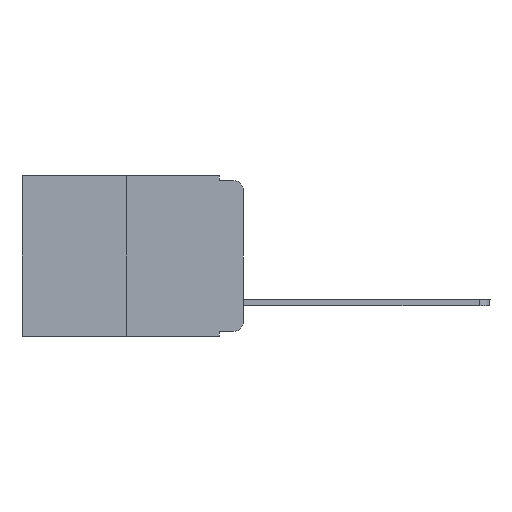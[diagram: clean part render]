
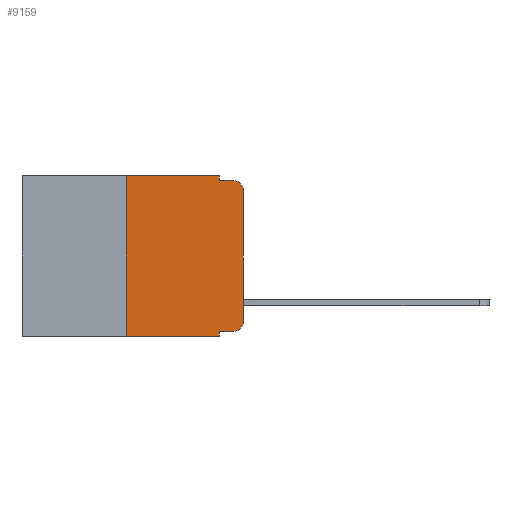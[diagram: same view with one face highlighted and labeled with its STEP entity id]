
A CAD part, left-side view. The second image highlights one B-rep face of the part: STEP entity #9159.
In plain terms, the highlighted planar face has unit normal (-1, 0, 0).
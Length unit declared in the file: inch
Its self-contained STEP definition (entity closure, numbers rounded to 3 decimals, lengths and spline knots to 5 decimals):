
#197 = LINE ( 'NONE', #9961, #6033 ) ;
#216 = DIRECTION ( 'NONE',  ( 0., 0., 1. ) ) ;
#510 = EDGE_CURVE ( 'NONE', #4199, #9617, #7737, .T. ) ;
#622 = PLANE ( 'NONE',  #2377 ) ;
#712 = CIRCLE ( 'NONE', #5788, 0.02 ) ;
#832 = CARTESIAN_POINT ( 'NONE',  ( 0., 0.473, 0. ) ) ;
#838 = LINE ( 'NONE', #6818, #10689 ) ;
#858 = DIRECTION ( 'NONE',  ( 0., -1., 0. ) ) ;
#878 = VECTOR ( 'NONE', #5546, 39.37008 ) ;
#1097 = EDGE_CURVE ( 'NONE', #9617, #4629, #4163, .T. ) ;
#1156 = CARTESIAN_POINT ( 'NONE',  ( 0., 0.02, -0.313 ) ) ;
#1245 = VECTOR ( 'NONE', #9817, 39.37008 ) ;
#1363 = DIRECTION ( 'NONE',  ( 0., 0., -1. ) ) ;
#1670 = DIRECTION ( 'NONE',  ( -1., 0., 0. ) ) ;
#2124 = EDGE_CURVE ( 'NONE', #9114, #5844, #5561, .T. ) ;
#2151 = CARTESIAN_POINT ( 'NONE',  ( 0., 0.051, -0.333 ) ) ;
#2206 = ORIENTED_EDGE ( 'NONE', *, *, #2124, .T. ) ;
#2251 = CARTESIAN_POINT ( 'NONE',  ( 0., 0.051, 0. ) ) ;
#2377 = AXIS2_PLACEMENT_3D ( 'NONE', #10420, #6311, #1363 ) ;
#2617 = ORIENTED_EDGE ( 'NONE', *, *, #9771, .T. ) ;
#2679 = CARTESIAN_POINT ( 'NONE',  ( 0., 0., -0.313 ) ) ;
#2784 = ORIENTED_EDGE ( 'NONE', *, *, #6930, .F. ) ;
#3306 = LINE ( 'NONE', #8320, #6009 ) ;
#3744 = DIRECTION ( 'NONE',  ( -1., 0., 0. ) ) ;
#4052 = ORIENTED_EDGE ( 'NONE', *, *, #8165, .T. ) ;
#4053 = VECTOR ( 'NONE', #10527, 39.37008 ) ;
#4152 = VECTOR ( 'NONE', #4890, 39.37008 ) ;
#4163 = LINE ( 'NONE', #9756, #4152 ) ;
#4199 = VERTEX_POINT ( 'NONE', #8731 ) ;
#4396 = ORIENTED_EDGE ( 'NONE', *, *, #1097, .F. ) ;
#4552 = ORIENTED_EDGE ( 'NONE', *, *, #9254, .F. ) ;
#4629 = VERTEX_POINT ( 'NONE', #7718 ) ;
#4722 = CARTESIAN_POINT ( 'NONE',  ( 0., 0.25, -0.343 ) ) ;
#4819 = CARTESIAN_POINT ( 'NONE',  ( 0., 0., -0.03 ) ) ;
#4890 = DIRECTION ( 'NONE',  ( 0., 0., -1. ) ) ;
#4948 = ORIENTED_EDGE ( 'NONE', *, *, #8625, .F. ) ;
#5010 = CARTESIAN_POINT ( 'NONE',  ( 0., 0.02, -0.03 ) ) ;
#5152 = DIRECTION ( 'NONE',  ( 0., -1., 0. ) ) ;
#5404 = VECTOR ( 'NONE', #5794, 39.37008 ) ;
#5480 = EDGE_CURVE ( 'NONE', #8730, #5530, #3306, .T. ) ;
#5530 = VERTEX_POINT ( 'NONE', #10038 ) ;
#5546 = DIRECTION ( 'NONE',  ( 0., 0., 1. ) ) ;
#5561 = LINE ( 'NONE', #7059, #878 ) ;
#5788 = AXIS2_PLACEMENT_3D ( 'NONE', #5010, #1670, #9972 ) ;
#5794 = DIRECTION ( 'NONE',  ( 0., -1., 0. ) ) ;
#5824 = ORIENTED_EDGE ( 'NONE', *, *, #9613, .T. ) ;
#5844 = VERTEX_POINT ( 'NONE', #4819 ) ;
#6009 = VECTOR ( 'NONE', #5152, 39.37008 ) ;
#6033 = VECTOR ( 'NONE', #858, 39.37008 ) ;
#6241 = ORIENTED_EDGE ( 'NONE', *, *, #510, .F. ) ;
#6311 = DIRECTION ( 'NONE',  ( 1., 0., 0. ) ) ;
#6318 = CARTESIAN_POINT ( 'NONE',  ( 0., 0.473, -0.343 ) ) ;
#6320 = CARTESIAN_POINT ( 'NONE',  ( 0., 0.02, -0.01 ) ) ;
#6750 = EDGE_LOOP ( 'NONE', ( #2206, #5824, #4552, #4396, #6241, #4948, #4052, #2784, #6813, #2617 ) ) ;
#6791 = LINE ( 'NONE', #2251, #4053 ) ;
#6813 = ORIENTED_EDGE ( 'NONE', *, *, #5480, .T. ) ;
#6818 = CARTESIAN_POINT ( 'NONE',  ( 0., 0.25, 0. ) ) ;
#6930 = EDGE_CURVE ( 'NONE', #8730, #8749, #6791, .T. ) ;
#6940 = FACE_OUTER_BOUND ( 'NONE', #6750, .T. ) ;
#7059 = CARTESIAN_POINT ( 'NONE',  ( 0., 0., 0. ) ) ;
#7466 = LINE ( 'NONE', #6318, #1245 ) ;
#7718 = CARTESIAN_POINT ( 'NONE',  ( 0., 0.051, -0.01 ) ) ;
#7737 = LINE ( 'NONE', #832, #5404 ) ;
#7952 = CARTESIAN_POINT ( 'NONE',  ( 0., 0.051, -0.343 ) ) ;
#8165 = EDGE_CURVE ( 'NONE', #10624, #8749, #7466, .T. ) ;
#8320 = CARTESIAN_POINT ( 'NONE',  ( 0., 0.051, -0.333 ) ) ;
#8625 = EDGE_CURVE ( 'NONE', #10624, #4199, #838, .T. ) ;
#8680 = VERTEX_POINT ( 'NONE', #6320 ) ;
#8730 = VERTEX_POINT ( 'NONE', #2151 ) ;
#8731 = CARTESIAN_POINT ( 'NONE',  ( 0., 0.25, 0. ) ) ;
#8749 = VERTEX_POINT ( 'NONE', #7952 ) ;
#9114 = VERTEX_POINT ( 'NONE', #2679 ) ;
#9135 = CARTESIAN_POINT ( 'NONE',  ( 0., 0.051, 0. ) ) ;
#9159 = ADVANCED_FACE ( 'NONE', ( #6940 ), #622, .F. ) ;
#9254 = EDGE_CURVE ( 'NONE', #4629, #8680, #197, .T. ) ;
#9507 = DIRECTION ( 'NONE',  ( 0., 0., -1. ) ) ;
#9613 = EDGE_CURVE ( 'NONE', #5844, #8680, #712, .T. ) ;
#9617 = VERTEX_POINT ( 'NONE', #9135 ) ;
#9756 = CARTESIAN_POINT ( 'NONE',  ( 0., 0.051, 0. ) ) ;
#9771 = EDGE_CURVE ( 'NONE', #5530, #9114, #9872, .T. ) ;
#9817 = DIRECTION ( 'NONE',  ( 0., -1., 0. ) ) ;
#9872 = CIRCLE ( 'NONE', #10464, 0.02 ) ;
#9961 = CARTESIAN_POINT ( 'NONE',  ( 0., 0.051, -0.01 ) ) ;
#9972 = DIRECTION ( 'NONE',  ( 0., 0., -1. ) ) ;
#10038 = CARTESIAN_POINT ( 'NONE',  ( 0., 0.02, -0.333 ) ) ;
#10420 = CARTESIAN_POINT ( 'NONE',  ( 0., 0.473, 0. ) ) ;
#10464 = AXIS2_PLACEMENT_3D ( 'NONE', #1156, #3744, #9507 ) ;
#10527 = DIRECTION ( 'NONE',  ( 0., 0., -1. ) ) ;
#10624 = VERTEX_POINT ( 'NONE', #4722 ) ;
#10689 = VECTOR ( 'NONE', #216, 39.37008 ) ;
